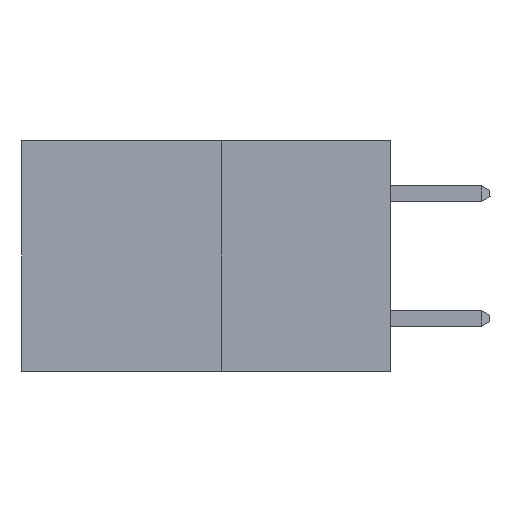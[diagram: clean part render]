
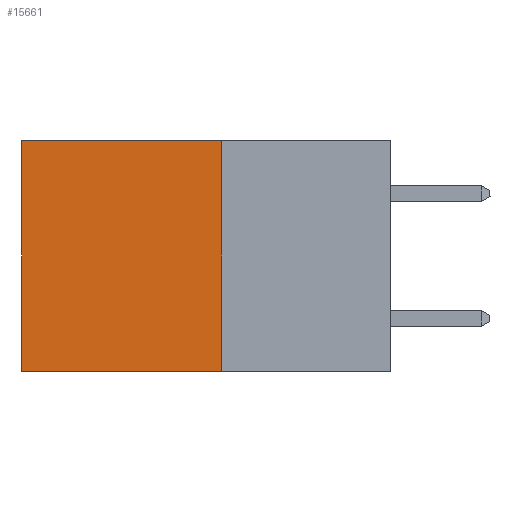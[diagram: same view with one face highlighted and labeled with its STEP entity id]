
A CAD part, left-side view. The second image highlights one B-rep face of the part: STEP entity #15661.
In plain terms, the highlighted planar face has unit normal (-1, 0, 0).
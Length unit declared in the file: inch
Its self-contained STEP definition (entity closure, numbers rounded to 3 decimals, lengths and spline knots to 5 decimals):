
#188 = LINE ( 'NONE', #11223, #8107 ) ;
#599 = CARTESIAN_POINT ( 'NONE',  ( 0.277, 0.59, -0.37 ) ) ;
#941 = VECTOR ( 'NONE', #7258, 39.37008 ) ;
#969 = VERTEX_POINT ( 'NONE', #9913 ) ;
#3322 = ORIENTED_EDGE ( 'NONE', *, *, #13353, .F. ) ;
#3506 = CARTESIAN_POINT ( 'NONE',  ( 0.277, 0.27, -0.37 ) ) ;
#4384 = VERTEX_POINT ( 'NONE', #14757 ) ;
#5760 = LINE ( 'NONE', #7039, #16544 ) ;
#6112 = LINE ( 'NONE', #8806, #941 ) ;
#7039 = CARTESIAN_POINT ( 'NONE',  ( 0.277, 0.27, -0.37 ) ) ;
#7258 = DIRECTION ( 'NONE',  ( 0., 1., 0. ) ) ;
#7452 = EDGE_CURVE ( 'NONE', #12821, #4384, #14948, .T. ) ;
#8107 = VECTOR ( 'NONE', #16988, 39.37008 ) ;
#8568 = DIRECTION ( 'NONE',  ( 0., 0., -1. ) ) ;
#8584 = DIRECTION ( 'NONE',  ( 1., 0., 0. ) ) ;
#8590 = CARTESIAN_POINT ( 'NONE',  ( 0.277, 0.27, -0.37 ) ) ;
#8747 = ORIENTED_EDGE ( 'NONE', *, *, #10864, .F. ) ;
#8806 = CARTESIAN_POINT ( 'NONE',  ( 0.277, 0.27, -0.37 ) ) ;
#8854 = PLANE ( 'NONE',  #12650 ) ;
#9555 = EDGE_LOOP ( 'NONE', ( #10377, #8747, #3322, #10119 ) ) ;
#9913 = CARTESIAN_POINT ( 'NONE',  ( 0.277, 0.27, 0. ) ) ;
#10119 = ORIENTED_EDGE ( 'NONE', *, *, #17713, .T. ) ;
#10377 = ORIENTED_EDGE ( 'NONE', *, *, #7452, .T. ) ;
#10864 = EDGE_CURVE ( 'NONE', #16177, #4384, #6112, .T. ) ;
#10911 = FACE_OUTER_BOUND ( 'NONE', #9555, .T. ) ;
#11223 = CARTESIAN_POINT ( 'NONE',  ( 0.277, 0.27, 0. ) ) ;
#12349 = DIRECTION ( 'NONE',  ( 0., 0., -1. ) ) ;
#12650 = AXIS2_PLACEMENT_3D ( 'NONE', #8590, #8584, #8568 ) ;
#12821 = VERTEX_POINT ( 'NONE', #13332 ) ;
#13332 = CARTESIAN_POINT ( 'NONE',  ( 0.277, 0.59, 0. ) ) ;
#13353 = EDGE_CURVE ( 'NONE', #969, #16177, #5760, .T. ) ;
#14316 = DIRECTION ( 'NONE',  ( 0., 0., -1. ) ) ;
#14757 = CARTESIAN_POINT ( 'NONE',  ( 0.277, 0.59, -0.37 ) ) ;
#14948 = LINE ( 'NONE', #599, #18317 ) ;
#15661 = ADVANCED_FACE ( 'NONE', ( #10911 ), #8854, .F. ) ;
#16177 = VERTEX_POINT ( 'NONE', #3506 ) ;
#16544 = VECTOR ( 'NONE', #14316, 39.37008 ) ;
#16988 = DIRECTION ( 'NONE',  ( 0., 1., 0. ) ) ;
#17713 = EDGE_CURVE ( 'NONE', #969, #12821, #188, .T. ) ;
#18317 = VECTOR ( 'NONE', #12349, 39.37008 ) ;
